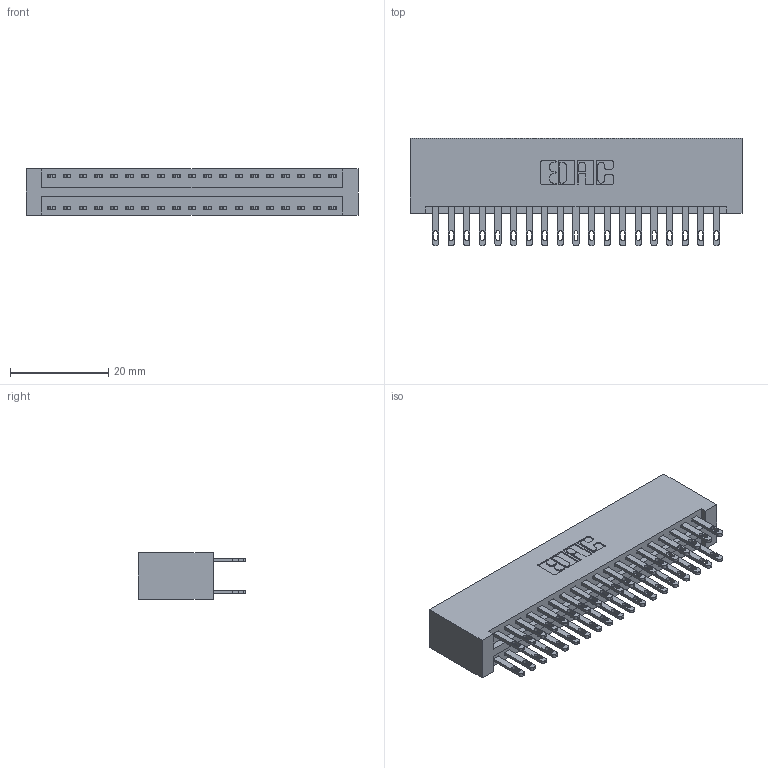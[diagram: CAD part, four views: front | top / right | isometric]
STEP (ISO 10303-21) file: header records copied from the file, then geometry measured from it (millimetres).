
FILE_DESCRIPTION (( 'STEP AP203' ), '1' );
FILE_NAME ('346-038-500-201.STEP', '2022-05-19T22:45:59', ( '' ), ( '' ), 'SwSTEP 2.0', 'SolidWorks 2020', '' );
FILE_SCHEMA (( 'CONFIG_CONTROL_DESIGN' ));
Length unit declared in the file: inch
Products named in the file (3): 346-038-500-201; 345-292-001_345-293-100; 346 Part_No Mounting Lugs
Assembly tree (39 placements, depth 2):
  346-038-500-201
    346 Part_No Mounting Lugs
    345-292-001_345-293-100  x38
Bounding box: 67.56 x 21.84 x 9.4 mm (x, y, z)
Volume: 7099.1 mm3; surface area: 9957.6 mm2
Topology: 39 solids, 39 shells, 1938 faces, 5891 edges, 3926 vertices
Faces by surface type: plane 1174, cylinder 764
Entity records: 15149 total; most frequent: CARTESIAN_POINT 2524, ORIENTED_EDGE 2458, DIRECTION 2273, EDGE_CURVE 1229, LINE 1025, VECTOR 1025, VERTEX_POINT 818, AXIS2_PLACEMENT_3D 624
